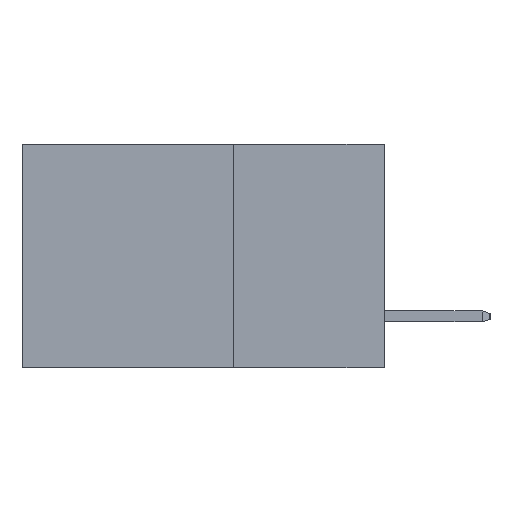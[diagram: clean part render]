
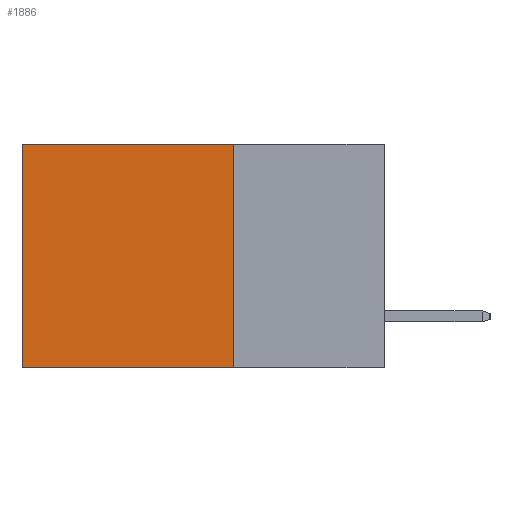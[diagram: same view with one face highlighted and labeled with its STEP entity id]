
A CAD part, left-side view. The second image highlights one B-rep face of the part: STEP entity #1886.
In plain terms, the highlighted planar face has unit normal (-1, 0, 0).
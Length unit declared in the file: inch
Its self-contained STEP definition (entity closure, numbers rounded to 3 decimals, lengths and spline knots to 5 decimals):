
#338 = EDGE_LOOP ( 'NONE', ( #8201, #11364, #1757, #9958 ) ) ;
#977 = VERTEX_POINT ( 'NONE', #6745 ) ;
#1634 = DIRECTION ( 'NONE',  ( 0., 0., -1. ) ) ;
#1690 = VERTEX_POINT ( 'NONE', #11350 ) ;
#1693 = CARTESIAN_POINT ( 'NONE',  ( 0.298, 0.6, 0. ) ) ;
#1757 = ORIENTED_EDGE ( 'NONE', *, *, #15804, .F. ) ;
#1886 = ADVANCED_FACE ( 'NONE', ( #7261 ), #7324, .F. ) ;
#2386 = LINE ( 'NONE', #10118, #6143 ) ;
#2555 = VERTEX_POINT ( 'NONE', #3286 ) ;
#3009 = DIRECTION ( 'NONE',  ( 0., 0., -1. ) ) ;
#3286 = CARTESIAN_POINT ( 'NONE',  ( 0.298, 0.25, -0.37 ) ) ;
#4400 = CARTESIAN_POINT ( 'NONE',  ( 0.298, 0.25, 0. ) ) ;
#5651 = DIRECTION ( 'NONE',  ( 0., 1., 0. ) ) ;
#6051 = DIRECTION ( 'NONE',  ( 1., 0., 0. ) ) ;
#6143 = VECTOR ( 'NONE', #6496, 39.37008 ) ;
#6210 = EDGE_CURVE ( 'NONE', #2555, #1690, #2386, .T. ) ;
#6388 = CARTESIAN_POINT ( 'NONE',  ( 0.298, 0.25, 0. ) ) ;
#6496 = DIRECTION ( 'NONE',  ( 0., 1., 0. ) ) ;
#6745 = CARTESIAN_POINT ( 'NONE',  ( 0.298, 0.25, 0. ) ) ;
#7261 = FACE_OUTER_BOUND ( 'NONE', #338, .T. ) ;
#7324 = PLANE ( 'NONE',  #11631 ) ;
#7763 = DIRECTION ( 'NONE',  ( 0., 0., -1. ) ) ;
#8201 = ORIENTED_EDGE ( 'NONE', *, *, #15837, .T. ) ;
#8946 = VECTOR ( 'NONE', #3009, 39.37008 ) ;
#9052 = CARTESIAN_POINT ( 'NONE',  ( 0.298, 0.25, 0. ) ) ;
#9375 = VECTOR ( 'NONE', #5651, 39.37008 ) ;
#9752 = LINE ( 'NONE', #4400, #9375 ) ;
#9958 = ORIENTED_EDGE ( 'NONE', *, *, #10588, .T. ) ;
#10118 = CARTESIAN_POINT ( 'NONE',  ( 0.298, 0.25, -0.37 ) ) ;
#10320 = CARTESIAN_POINT ( 'NONE',  ( 0.298, 0.6, 0. ) ) ;
#10418 = VECTOR ( 'NONE', #1634, 39.37008 ) ;
#10588 = EDGE_CURVE ( 'NONE', #977, #12968, #9752, .T. ) ;
#11350 = CARTESIAN_POINT ( 'NONE',  ( 0.298, 0.6, -0.37 ) ) ;
#11364 = ORIENTED_EDGE ( 'NONE', *, *, #6210, .F. ) ;
#11631 = AXIS2_PLACEMENT_3D ( 'NONE', #6388, #6051, #7763 ) ;
#12471 = LINE ( 'NONE', #1693, #8946 ) ;
#12816 = LINE ( 'NONE', #9052, #10418 ) ;
#12968 = VERTEX_POINT ( 'NONE', #10320 ) ;
#15804 = EDGE_CURVE ( 'NONE', #977, #2555, #12816, .T. ) ;
#15837 = EDGE_CURVE ( 'NONE', #12968, #1690, #12471, .T. ) ;
